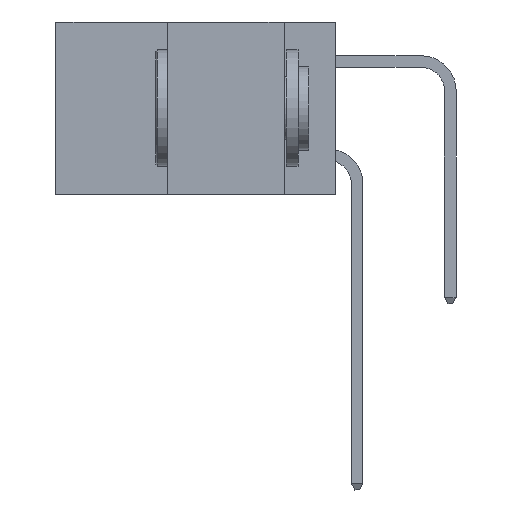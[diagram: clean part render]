
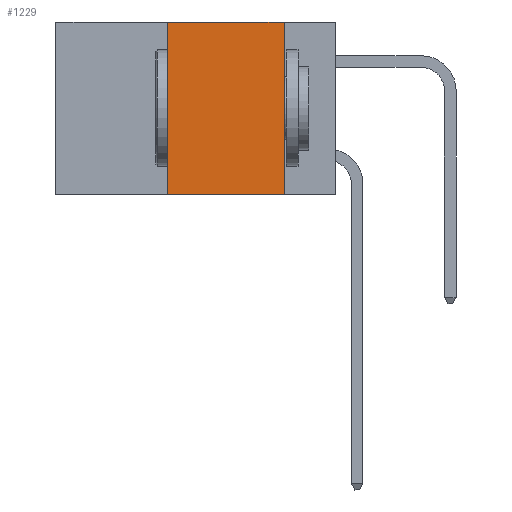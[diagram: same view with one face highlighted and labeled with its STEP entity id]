
A CAD part, left-side view. The second image highlights one B-rep face of the part: STEP entity #1229.
In plain terms, the highlighted planar face has unit normal (-1, 0, 0).
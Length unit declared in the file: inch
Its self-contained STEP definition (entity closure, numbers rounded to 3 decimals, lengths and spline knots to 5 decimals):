
#815 = CARTESIAN_POINT ( 'NONE',  ( 0., 0.11, 0. ) ) ;
#1229 = ADVANCED_FACE ( 'NONE', ( #22053 ), #15584, .F. ) ;
#1234 = CARTESIAN_POINT ( 'NONE',  ( 0., 0.11, 0. ) ) ;
#2375 = LINE ( 'NONE', #20295, #18559 ) ;
#2533 = VERTEX_POINT ( 'NONE', #21122 ) ;
#2994 = LINE ( 'NONE', #8338, #22682 ) ;
#4527 = ORIENTED_EDGE ( 'NONE', *, *, #10606, .F. ) ;
#6458 = VERTEX_POINT ( 'NONE', #11221 ) ;
#8338 = CARTESIAN_POINT ( 'NONE',  ( 0., 0.6, 0. ) ) ;
#9639 = DIRECTION ( 'NONE',  ( 0., 0., -1. ) ) ;
#9931 = DIRECTION ( 'NONE',  ( 0., 0., 1. ) ) ;
#10375 = AXIS2_PLACEMENT_3D ( 'NONE', #21628, #23645, #9639 ) ;
#10594 = VECTOR ( 'NONE', #11487, 39.37008 ) ;
#10606 = EDGE_CURVE ( 'NONE', #2533, #11942, #2375, .T. ) ;
#10623 = ORIENTED_EDGE ( 'NONE', *, *, #12104, .T. ) ;
#11221 = CARTESIAN_POINT ( 'NONE',  ( 0., 0.11, -0.37 ) ) ;
#11402 = DIRECTION ( 'NONE',  ( 0., -1., 0. ) ) ;
#11487 = DIRECTION ( 'NONE',  ( 0., -1., 0. ) ) ;
#11551 = DIRECTION ( 'NONE',  ( 0., 0., -1. ) ) ;
#11942 = VERTEX_POINT ( 'NONE', #14435 ) ;
#12023 = EDGE_CURVE ( 'NONE', #11942, #14712, #2994, .T. ) ;
#12104 = EDGE_CURVE ( 'NONE', #2533, #6458, #17898, .T. ) ;
#13156 = VECTOR ( 'NONE', #11551, 39.37008 ) ;
#14435 = CARTESIAN_POINT ( 'NONE',  ( 0., 0.36, 0. ) ) ;
#14712 = VERTEX_POINT ( 'NONE', #1234 ) ;
#15393 = LINE ( 'NONE', #815, #13156 ) ;
#15584 = PLANE ( 'NONE',  #10375 ) ;
#17796 = ORIENTED_EDGE ( 'NONE', *, *, #12023, .F. ) ;
#17898 = LINE ( 'NONE', #23550, #10594 ) ;
#18153 = EDGE_LOOP ( 'NONE', ( #25248, #17796, #4527, #10623 ) ) ;
#18559 = VECTOR ( 'NONE', #9931, 39.37008 ) ;
#20295 = CARTESIAN_POINT ( 'NONE',  ( 0., 0.36, 0. ) ) ;
#21122 = CARTESIAN_POINT ( 'NONE',  ( 0., 0.36, -0.37 ) ) ;
#21628 = CARTESIAN_POINT ( 'NONE',  ( 0., 0.6, 0. ) ) ;
#22006 = EDGE_CURVE ( 'NONE', #14712, #6458, #15393, .T. ) ;
#22053 = FACE_OUTER_BOUND ( 'NONE', #18153, .T. ) ;
#22682 = VECTOR ( 'NONE', #11402, 39.37008 ) ;
#23550 = CARTESIAN_POINT ( 'NONE',  ( 0., 0.6, -0.37 ) ) ;
#23645 = DIRECTION ( 'NONE',  ( 1., 0., 0. ) ) ;
#25248 = ORIENTED_EDGE ( 'NONE', *, *, #22006, .F. ) ;
